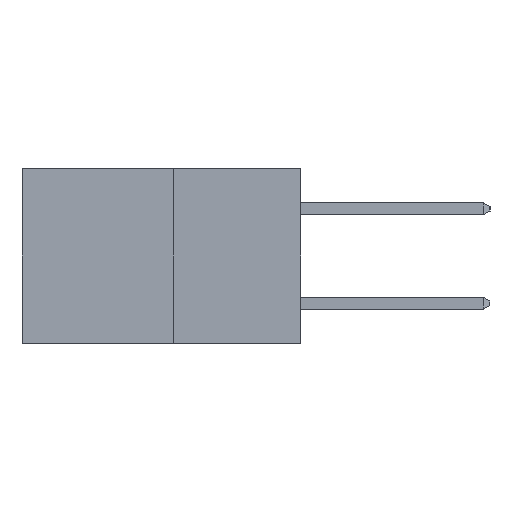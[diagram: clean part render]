
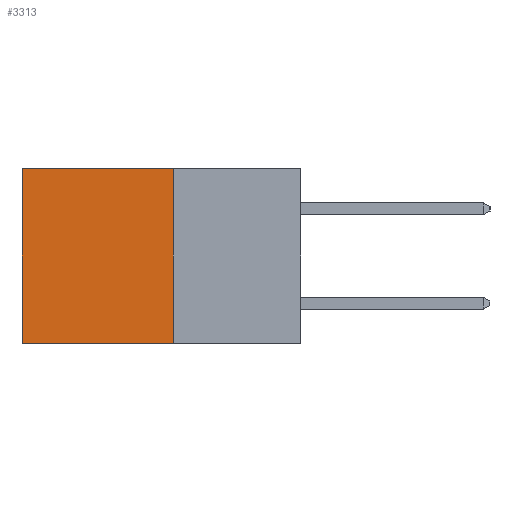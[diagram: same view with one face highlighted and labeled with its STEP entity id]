
A CAD part, left-side view. The second image highlights one B-rep face of the part: STEP entity #3313.
In plain terms, the highlighted planar face has unit normal (-1, 0, 0).
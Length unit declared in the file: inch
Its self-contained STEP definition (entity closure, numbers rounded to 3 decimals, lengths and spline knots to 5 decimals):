
#473 = ORIENTED_EDGE ( 'NONE', *, *, #982, .F. ) ;
#816 = ORIENTED_EDGE ( 'NONE', *, *, #8012, .F. ) ;
#982 = EDGE_CURVE ( 'NONE', #6478, #1901, #1519, .T. ) ;
#1519 = LINE ( 'NONE', #5923, #8883 ) ;
#1865 = CARTESIAN_POINT ( 'NONE',  ( 0.277, 0.59, 0. ) ) ;
#1901 = VERTEX_POINT ( 'NONE', #2091 ) ;
#2013 = LINE ( 'NONE', #11802, #6617 ) ;
#2091 = CARTESIAN_POINT ( 'NONE',  ( 0.277, 0.27, -0.37 ) ) ;
#2470 = ORIENTED_EDGE ( 'NONE', *, *, #3028, .T. ) ;
#2696 = ORIENTED_EDGE ( 'NONE', *, *, #9929, .T. ) ;
#3028 = EDGE_CURVE ( 'NONE', #10714, #11876, #9535, .T. ) ;
#3313 = ADVANCED_FACE ( 'NONE', ( #6656 ), #8502, .F. ) ;
#3418 = VECTOR ( 'NONE', #5374, 39.37008 ) ;
#3804 = DIRECTION ( 'NONE',  ( 0., 0., -1. ) ) ;
#4391 = CARTESIAN_POINT ( 'NONE',  ( 0.277, 0.27, -0.37 ) ) ;
#5374 = DIRECTION ( 'NONE',  ( 0., 1., 0. ) ) ;
#5923 = CARTESIAN_POINT ( 'NONE',  ( 0.277, 0.27, -0.37 ) ) ;
#6027 = DIRECTION ( 'NONE',  ( 0., 0., -1. ) ) ;
#6478 = VERTEX_POINT ( 'NONE', #7966 ) ;
#6617 = VECTOR ( 'NONE', #7178, 39.37008 ) ;
#6656 = FACE_OUTER_BOUND ( 'NONE', #10639, .T. ) ;
#6807 = VECTOR ( 'NONE', #3804, 39.37008 ) ;
#7178 = DIRECTION ( 'NONE',  ( 0., 1., 0. ) ) ;
#7966 = CARTESIAN_POINT ( 'NONE',  ( 0.277, 0.27, 0. ) ) ;
#8012 = EDGE_CURVE ( 'NONE', #1901, #11876, #10399, .T. ) ;
#8502 = PLANE ( 'NONE',  #8856 ) ;
#8856 = AXIS2_PLACEMENT_3D ( 'NONE', #9510, #11375, #6027 ) ;
#8883 = VECTOR ( 'NONE', #10870, 39.37008 ) ;
#9121 = CARTESIAN_POINT ( 'NONE',  ( 0.277, 0.59, -0.37 ) ) ;
#9510 = CARTESIAN_POINT ( 'NONE',  ( 0.277, 0.27, -0.37 ) ) ;
#9535 = LINE ( 'NONE', #10862, #6807 ) ;
#9929 = EDGE_CURVE ( 'NONE', #6478, #10714, #2013, .T. ) ;
#10399 = LINE ( 'NONE', #4391, #3418 ) ;
#10639 = EDGE_LOOP ( 'NONE', ( #2470, #816, #473, #2696 ) ) ;
#10714 = VERTEX_POINT ( 'NONE', #1865 ) ;
#10862 = CARTESIAN_POINT ( 'NONE',  ( 0.277, 0.59, -0.37 ) ) ;
#10870 = DIRECTION ( 'NONE',  ( 0., 0., -1. ) ) ;
#11375 = DIRECTION ( 'NONE',  ( 1., 0., 0. ) ) ;
#11802 = CARTESIAN_POINT ( 'NONE',  ( 0.277, 0.27, 0. ) ) ;
#11876 = VERTEX_POINT ( 'NONE', #9121 ) ;
